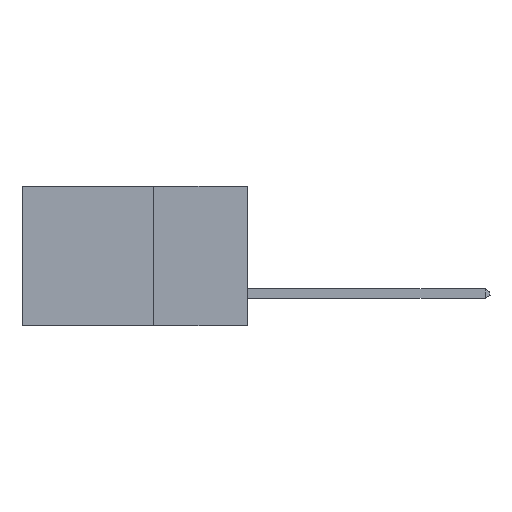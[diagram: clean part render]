
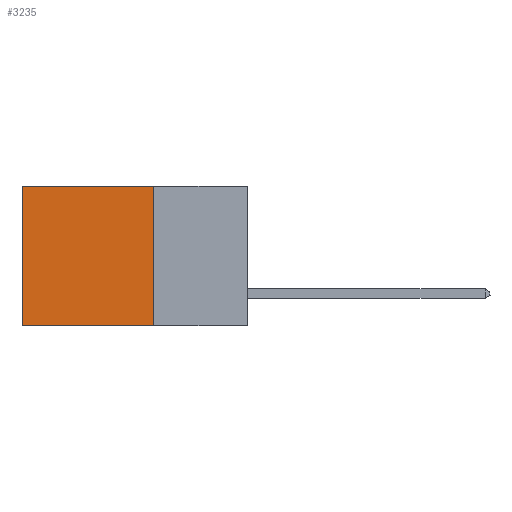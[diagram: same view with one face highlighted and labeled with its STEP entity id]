
A CAD part, left-side view. The second image highlights one B-rep face of the part: STEP entity #3235.
In plain terms, the highlighted planar face has unit normal (-1, 0, 0).
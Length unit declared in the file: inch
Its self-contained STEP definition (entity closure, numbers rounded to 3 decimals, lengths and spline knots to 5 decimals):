
#56 = EDGE_CURVE ( 'NONE', #1368, #3707, #1907, .T. ) ;
#146 = CARTESIAN_POINT ( 'NONE',  ( 0.298, 0.25, 0. ) ) ;
#157 = AXIS2_PLACEMENT_3D ( 'NONE', #2848, #3844, #5974 ) ;
#818 = VECTOR ( 'NONE', #11456, 39.37008 ) ;
#903 = EDGE_CURVE ( 'NONE', #1368, #3449, #1875, .T. ) ;
#1240 = EDGE_CURVE ( 'NONE', #3707, #3703, #11373, .T. ) ;
#1368 = VERTEX_POINT ( 'NONE', #12606 ) ;
#1697 = PLANE ( 'NONE',  #157 ) ;
#1875 = LINE ( 'NONE', #1912, #7142 ) ;
#1907 = LINE ( 'NONE', #146, #13920 ) ;
#1912 = CARTESIAN_POINT ( 'NONE',  ( 0.298, 0.25, 0. ) ) ;
#2548 = ORIENTED_EDGE ( 'NONE', *, *, #1240, .T. ) ;
#2740 = CARTESIAN_POINT ( 'NONE',  ( 0.298, 0.6, 0. ) ) ;
#2796 = ORIENTED_EDGE ( 'NONE', *, *, #56, .T. ) ;
#2848 = CARTESIAN_POINT ( 'NONE',  ( 0.298, 0.25, 0. ) ) ;
#3235 = ADVANCED_FACE ( 'NONE', ( #11460 ), #1697, .F. ) ;
#3367 = LINE ( 'NONE', #12738, #818 ) ;
#3449 = VERTEX_POINT ( 'NONE', #12892 ) ;
#3703 = VERTEX_POINT ( 'NONE', #8005 ) ;
#3707 = VERTEX_POINT ( 'NONE', #12333 ) ;
#3844 = DIRECTION ( 'NONE',  ( 1., 0., 0. ) ) ;
#4953 = DIRECTION ( 'NONE',  ( 0., 0., -1. ) ) ;
#5350 = ORIENTED_EDGE ( 'NONE', *, *, #11004, .F. ) ;
#5974 = DIRECTION ( 'NONE',  ( 0., 0., -1. ) ) ;
#7142 = VECTOR ( 'NONE', #9505, 39.37008 ) ;
#7191 = ORIENTED_EDGE ( 'NONE', *, *, #903, .F. ) ;
#7721 = DIRECTION ( 'NONE',  ( 0., 1., 0. ) ) ;
#7851 = VECTOR ( 'NONE', #4953, 39.37008 ) ;
#8005 = CARTESIAN_POINT ( 'NONE',  ( 0.298, 0.6, -0.37 ) ) ;
#9505 = DIRECTION ( 'NONE',  ( 0., 0., -1. ) ) ;
#11004 = EDGE_CURVE ( 'NONE', #3449, #3703, #3367, .T. ) ;
#11373 = LINE ( 'NONE', #2740, #7851 ) ;
#11456 = DIRECTION ( 'NONE',  ( 0., 1., 0. ) ) ;
#11460 = FACE_OUTER_BOUND ( 'NONE', #12022, .T. ) ;
#12022 = EDGE_LOOP ( 'NONE', ( #2548, #5350, #7191, #2796 ) ) ;
#12333 = CARTESIAN_POINT ( 'NONE',  ( 0.298, 0.6, 0. ) ) ;
#12606 = CARTESIAN_POINT ( 'NONE',  ( 0.298, 0.25, 0. ) ) ;
#12738 = CARTESIAN_POINT ( 'NONE',  ( 0.298, 0.25, -0.37 ) ) ;
#12892 = CARTESIAN_POINT ( 'NONE',  ( 0.298, 0.25, -0.37 ) ) ;
#13920 = VECTOR ( 'NONE', #7721, 39.37008 ) ;
